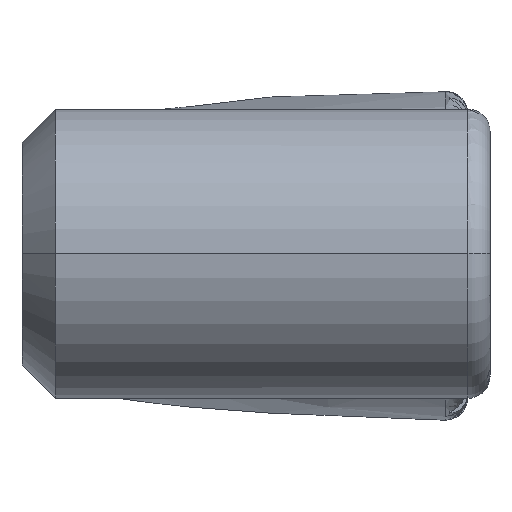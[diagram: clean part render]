
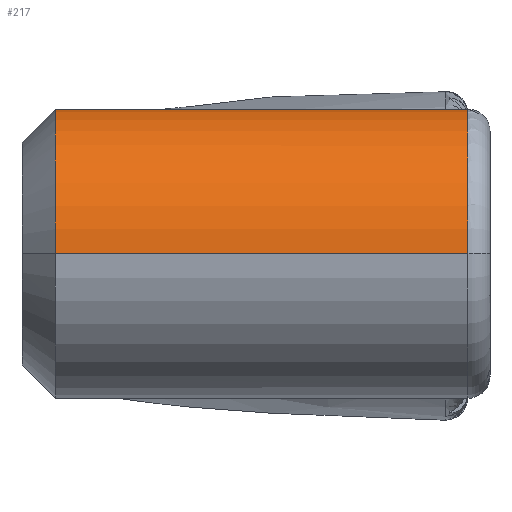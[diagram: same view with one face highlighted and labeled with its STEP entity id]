
A CAD part, top view. The second image highlights one B-rep face of the part: STEP entity #217.
In plain terms, the highlighted cylindrical face has radius 6.5 mm (diameter 13 mm), a partial arc.
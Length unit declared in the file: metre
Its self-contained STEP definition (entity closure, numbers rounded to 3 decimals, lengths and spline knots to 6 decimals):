
#217=ADVANCED_FACE('0:62371',(#592),#593,.T.);
#592=FACE_OUTER_BOUND('',#1139,.T.);
#593=CYLINDRICAL_SURFACE('',#1140,0.0065);
#1139=EDGE_LOOP('',(#2887,#2888,#2889,#2890,#2891,#2892));
#1140=AXIS2_PLACEMENT_3D('',#2893,#2894,#2895);
#2887=ORIENTED_EDGE('',*,*,#3135,.T.);
#2888=ORIENTED_EDGE('',*,*,#3560,.F.);
#2889=ORIENTED_EDGE('',*,*,#3141,.F.);
#2890=ORIENTED_EDGE('',*,*,#3558,.F.);
#2891=ORIENTED_EDGE('',*,*,#3559,.F.);
#2892=ORIENTED_EDGE('',*,*,#3116,.F.);
#2893=CARTESIAN_POINT('',(0.075679,0.047829,-0.020721));
#2894=DIRECTION('',(1.0,0.,0.));
#2895=DIRECTION('',(0.,0.,-1.0));
#3116=EDGE_CURVE('0:63727',#3660,#3663,#3664,.F.);
#3135=EDGE_CURVE('',#3660,#3623,#3696,.T.);
#3141=EDGE_CURVE('0:63703',#3704,#3706,#3707,.F.);
#3558=EDGE_CURVE('0:63703',#4390,#3704,#4392,.F.);
#3559=EDGE_CURVE('0:63715',#3663,#4390,#4393,.T.);
#3560=EDGE_CURVE('0:63724',#3706,#3623,#4394,.T.);
#3623=VERTEX_POINT('',#4473);
#3660=VERTEX_POINT('',#4538);
#3663=VERTEX_POINT('',#4542);
#3664=CIRCLE('',#4543,0.0065);
#3696=LINE('',#4618,#4619);
#3704=VERTEX_POINT('',#4652);
#3706=VERTEX_POINT('',#4655);
#3707=B_SPLINE_CURVE_WITH_KNOTS('',3,(#4656,#4657,#4658,#4659,#4660,#4661,#4662,#4663,#4664,#4665,#4666,#4667,#4668),.UNSPECIFIED.,.F.,.F.,(4,3,3,3,4),(0.152527,0.206541,0.236016,0.285993,0.308275),.UNSPECIFIED.);
#4390=VERTEX_POINT('',#6278);
#4392=B_SPLINE_CURVE_WITH_KNOTS('',3,(#6281,#6282,#6283,#6284,#6285,#6286,#6287,#6288,#6289,#6290,#6291,#6292,#6293),.UNSPECIFIED.,.F.,.F.,(4,3,3,3,4),(0.152527,0.206541,0.236016,0.285993,0.308275),.UNSPECIFIED.);
#4393=LINE('',#6294,#6295);
#4394=CIRCLE('',#6296,0.0065);
#4473=CARTESIAN_POINT('',(0.080679,0.047829,-0.014221));
#4538=CARTESIAN_POINT('',(0.062179,0.047829,-0.014221));
#4542=CARTESIAN_POINT('',(0.062179,0.050629,-0.026587));
#4543=AXIS2_PLACEMENT_3D('',#6548,#6549,#6550);
#4618=CARTESIAN_POINT('',(0.075679,0.047829,-0.014221));
#4619=VECTOR('',#6585,1.0);
#4652=CARTESIAN_POINT('',(0.080386,0.050337,-0.026718));
#4655=CARTESIAN_POINT('',(0.080679,0.049629,-0.026966));
#4656=CARTESIAN_POINT('',(0.080679,0.049629,-0.026966));
#4657=CARTESIAN_POINT('',(0.080679,0.049802,-0.026917));
#4658=CARTESIAN_POINT('',(0.08063,0.049988,-0.026854));
#4659=CARTESIAN_POINT('',(0.080537,0.050144,-0.026795));
#4660=CARTESIAN_POINT('',(0.080486,0.050228,-0.026763));
#4661=CARTESIAN_POINT('',(0.080425,0.050303,-0.026732));
#4662=CARTESIAN_POINT('',(0.080354,0.050367,-0.026705));
#4663=CARTESIAN_POINT('',(0.080234,0.050477,-0.026658));
#4664=CARTESIAN_POINT('',(0.080074,0.050564,-0.026618));
#4665=CARTESIAN_POINT('',(0.079905,0.050604,-0.026599));
#4666=CARTESIAN_POINT('',(0.07983,0.050621,-0.026591));
#4667=CARTESIAN_POINT('',(0.079753,0.050629,-0.026587));
#4668=CARTESIAN_POINT('',(0.079679,0.050629,-0.026587));
#6278=CARTESIAN_POINT('',(0.079679,0.050629,-0.026587));
#6281=CARTESIAN_POINT('',(0.080679,0.049629,-0.026966));
#6282=CARTESIAN_POINT('',(0.080679,0.049802,-0.026917));
#6283=CARTESIAN_POINT('',(0.08063,0.049988,-0.026854));
#6284=CARTESIAN_POINT('',(0.080537,0.050144,-0.026795));
#6285=CARTESIAN_POINT('',(0.080486,0.050228,-0.026763));
#6286=CARTESIAN_POINT('',(0.080425,0.050303,-0.026732));
#6287=CARTESIAN_POINT('',(0.080354,0.050367,-0.026705));
#6288=CARTESIAN_POINT('',(0.080234,0.050477,-0.026658));
#6289=CARTESIAN_POINT('',(0.080074,0.050564,-0.026618));
#6290=CARTESIAN_POINT('',(0.079905,0.050604,-0.026599));
#6291=CARTESIAN_POINT('',(0.07983,0.050621,-0.026591));
#6292=CARTESIAN_POINT('',(0.079753,0.050629,-0.026587));
#6293=CARTESIAN_POINT('',(0.079679,0.050629,-0.026587));
#6294=CARTESIAN_POINT('',(0.075679,0.050629,-0.026587));
#6295=VECTOR('',#7032,0.0175);
#6296=AXIS2_PLACEMENT_3D('',#7033,#7034,#7035);
#6548=CARTESIAN_POINT('',(0.062179,0.047829,-0.020721));
#6549=DIRECTION('',(1.0,0.,0.));
#6550=DIRECTION('',(0.,0.,-1.0));
#6585=DIRECTION('',(1.0,0.,0.));
#7032=DIRECTION('',(1.0,0.,0.));
#7033=CARTESIAN_POINT('',(0.080679,0.047829,-0.020721));
#7034=DIRECTION('',(1.0,0.,0.));
#7035=DIRECTION('',(0.,0.,-1.0));
